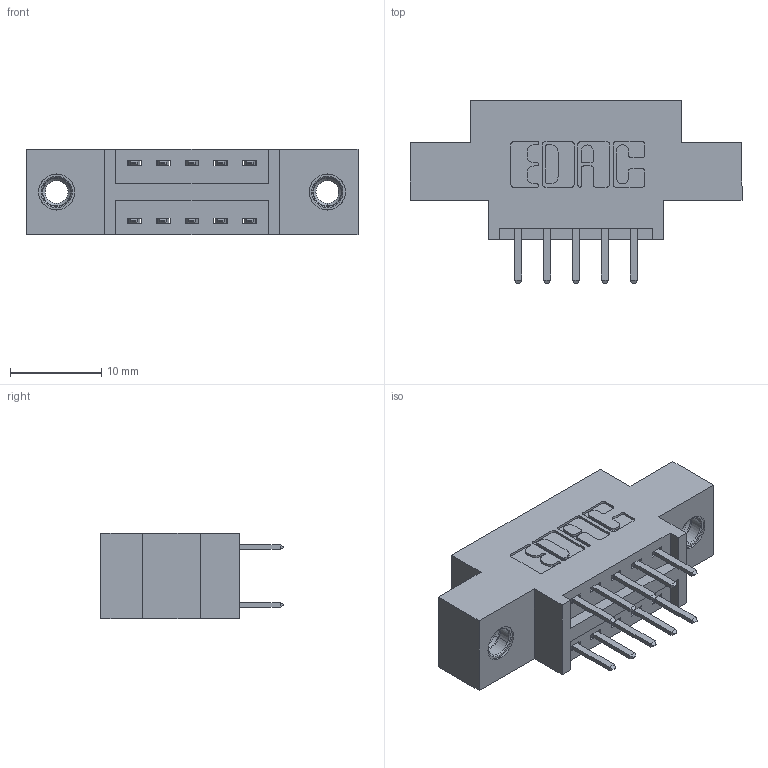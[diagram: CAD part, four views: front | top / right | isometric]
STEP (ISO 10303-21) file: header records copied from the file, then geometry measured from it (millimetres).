
FILE_DESCRIPTION (( 'STEP AP203' ), '1' );
FILE_NAME ('396-010-520-807.STEP', '2019-11-01T16:38:51', ( '' ), ( '' ), 'SwSTEP 2.0', 'SolidWorks 2016', '' );
FILE_SCHEMA (( 'CONFIG_CONTROL_DESIGN' ));
Length unit declared in the file: inch
Products named in the file (4): 346 Part_0.170 Offset - 0.156 Dia-TI; 345-292-001_345-293-120; 345-250-001_345-250-005-103; 396-010-520-807
Assembly tree (13 placements, depth 2):
  396-010-520-807
    346 Part_0.170 Offset - 0.156 Dia-TI
    345-292-001_345-293-120  x10
    345-250-001_345-250-005-103  x2
Bounding box: 36.45 x 20.02 x 9.4 mm (x, y, z)
Volume: 3094.3 mm3; surface area: 3874.9 mm2
Topology: 13 solids, 13 shells, 746 faces, 2107 edges, 1370 vertices
Faces by surface type: plane 482, cylinder 248, cone 12, torus 4
Entity records: 9676 total; most frequent: CARTESIAN_POINT 1643, ORIENTED_EDGE 1558, DIRECTION 1513, EDGE_CURVE 779, VECTOR 603, LINE 603, VERTEX_POINT 512, AXIS2_PLACEMENT_3D 455
